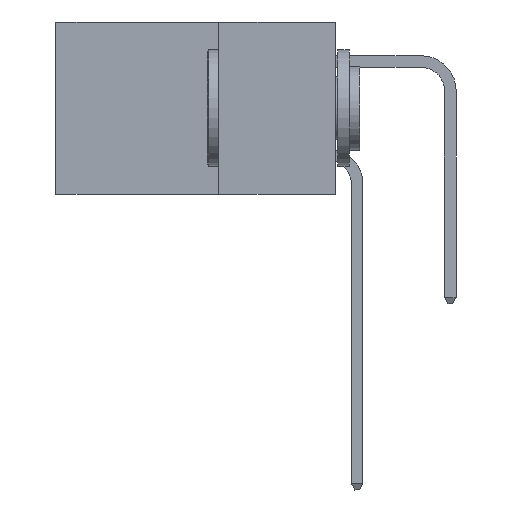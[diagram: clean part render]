
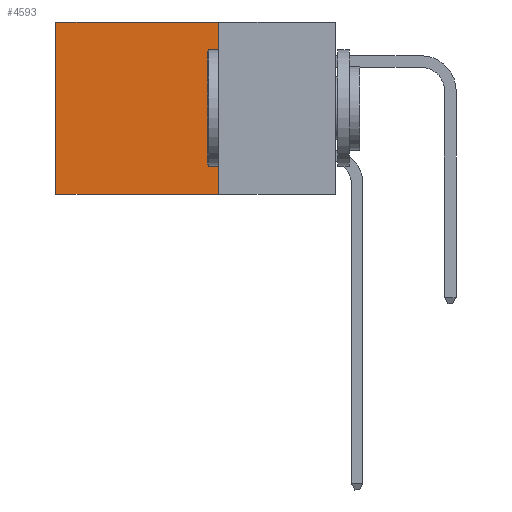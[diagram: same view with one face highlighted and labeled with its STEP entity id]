
A CAD part, left-side view. The second image highlights one B-rep face of the part: STEP entity #4593.
In plain terms, the highlighted planar face has unit normal (-1, 0, 0).
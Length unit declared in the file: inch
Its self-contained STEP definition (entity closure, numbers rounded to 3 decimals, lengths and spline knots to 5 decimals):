
#125 = LINE ( 'NONE', #25616, #18261 ) ;
#704 = CARTESIAN_POINT ( 'NONE',  ( 0.2875, 0.6, -0.37 ) ) ;
#1911 = DIRECTION ( 'NONE',  ( 1., 0., 0. ) ) ;
#1970 = DIRECTION ( 'NONE',  ( 0., 1., 0. ) ) ;
#2211 = LINE ( 'NONE', #19770, #26184 ) ;
#2732 = EDGE_CURVE ( 'NONE', #6935, #23444, #26139, .T. ) ;
#3433 = CARTESIAN_POINT ( 'NONE',  ( 0.2875, 0.6, 0. ) ) ;
#3831 = ORIENTED_EDGE ( 'NONE', *, *, #22618, .T. ) ;
#4593 = ADVANCED_FACE ( 'NONE', ( #12975 ), #6478, .F. ) ;
#6478 = PLANE ( 'NONE',  #8071 ) ;
#6488 = VECTOR ( 'NONE', #1970, 39.37008 ) ;
#6839 = DIRECTION ( 'NONE',  ( 0., 1., 0. ) ) ;
#6935 = VERTEX_POINT ( 'NONE', #19902 ) ;
#8071 = AXIS2_PLACEMENT_3D ( 'NONE', #11022, #1911, #27404 ) ;
#8656 = LINE ( 'NONE', #29607, #6488 ) ;
#8872 = EDGE_CURVE ( 'NONE', #20121, #23444, #8656, .T. ) ;
#10398 = DIRECTION ( 'NONE',  ( 0., 0., -1. ) ) ;
#11022 = CARTESIAN_POINT ( 'NONE',  ( 0.2875, 0.25, 0. ) ) ;
#12295 = ORIENTED_EDGE ( 'NONE', *, *, #2732, .T. ) ;
#12958 = ORIENTED_EDGE ( 'NONE', *, *, #18549, .F. ) ;
#12975 = FACE_OUTER_BOUND ( 'NONE', #21736, .T. ) ;
#17531 = DIRECTION ( 'NONE',  ( 0., 0., -1. ) ) ;
#18261 = VECTOR ( 'NONE', #6839, 39.37008 ) ;
#18549 = EDGE_CURVE ( 'NONE', #22795, #20121, #2211, .T. ) ;
#19770 = CARTESIAN_POINT ( 'NONE',  ( 0.2875, 0.25, 0. ) ) ;
#19902 = CARTESIAN_POINT ( 'NONE',  ( 0.2875, 0.6, 0. ) ) ;
#20121 = VERTEX_POINT ( 'NONE', #26191 ) ;
#21736 = EDGE_LOOP ( 'NONE', ( #12295, #28214, #12958, #3831 ) ) ;
#22618 = EDGE_CURVE ( 'NONE', #22795, #6935, #125, .T. ) ;
#22795 = VERTEX_POINT ( 'NONE', #23764 ) ;
#23444 = VERTEX_POINT ( 'NONE', #704 ) ;
#23764 = CARTESIAN_POINT ( 'NONE',  ( 0.2875, 0.25, 0. ) ) ;
#25071 = VECTOR ( 'NONE', #10398, 39.37008 ) ;
#25616 = CARTESIAN_POINT ( 'NONE',  ( 0.2875, 0.25, 0. ) ) ;
#26139 = LINE ( 'NONE', #3433, #25071 ) ;
#26184 = VECTOR ( 'NONE', #17531, 39.37008 ) ;
#26191 = CARTESIAN_POINT ( 'NONE',  ( 0.2875, 0.25, -0.37 ) ) ;
#27404 = DIRECTION ( 'NONE',  ( 0., 0., -1. ) ) ;
#28214 = ORIENTED_EDGE ( 'NONE', *, *, #8872, .F. ) ;
#29607 = CARTESIAN_POINT ( 'NONE',  ( 0.2875, 0.25, -0.37 ) ) ;
